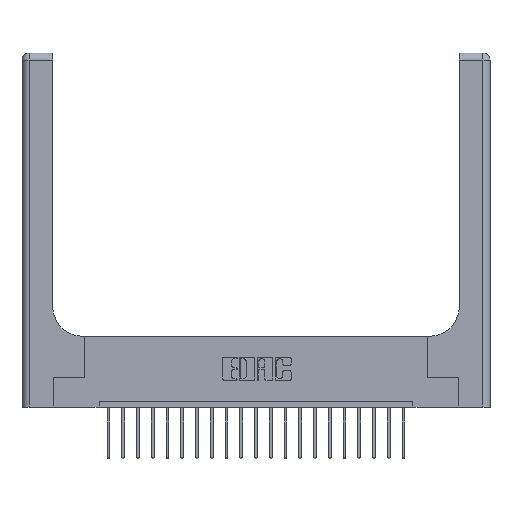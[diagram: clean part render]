
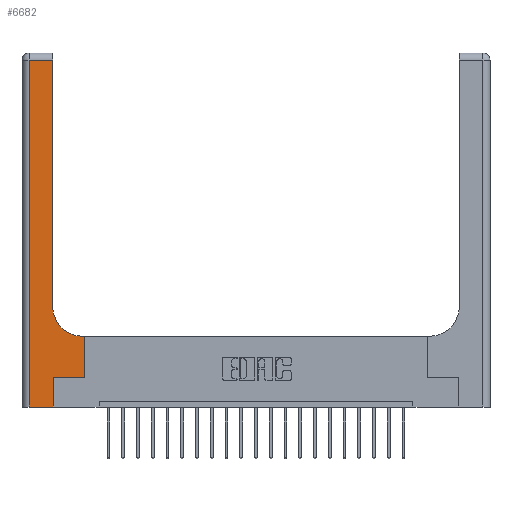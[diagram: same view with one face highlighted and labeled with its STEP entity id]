
A CAD part, top view. The second image highlights one B-rep face of the part: STEP entity #6682.
In plain terms, the highlighted planar face has unit normal (0, 0, 1).
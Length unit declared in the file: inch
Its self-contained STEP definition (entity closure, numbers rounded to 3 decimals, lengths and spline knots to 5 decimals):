
#1258 = DIRECTION ( 'NONE',  ( 0., 0., -1. ) ) ;
#1287 = EDGE_CURVE ( 'NONE', #20009, #4010, #11198, .T. ) ;
#1305 = VERTEX_POINT ( 'NONE', #16613 ) ;
#1809 = EDGE_CURVE ( 'NONE', #7656, #2058, #10814, .T. ) ;
#2058 = VERTEX_POINT ( 'NONE', #15242 ) ;
#2691 = PLANE ( 'NONE',  #3644 ) ;
#2785 = ORIENTED_EDGE ( 'NONE', *, *, #13702, .T. ) ;
#3242 = DIRECTION ( 'NONE',  ( 0., -1., 0. ) ) ;
#3540 = CARTESIAN_POINT ( 'NONE',  ( 0.265, 0.25, 0.37 ) ) ;
#3644 = AXIS2_PLACEMENT_3D ( 'NONE', #16156, #1258, #12577 ) ;
#4010 = VERTEX_POINT ( 'NONE', #3540 ) ;
#4066 = VECTOR ( 'NONE', #6361, 39.37008 ) ;
#4165 = CARTESIAN_POINT ( 'NONE',  ( 0.265, 0.25, 0.37 ) ) ;
#4568 = CARTESIAN_POINT ( 'NONE',  ( 0., 0., 0.37 ) ) ;
#4676 = LINE ( 'NONE', #4568, #19640 ) ;
#4828 = EDGE_CURVE ( 'NONE', #13716, #13617, #13362, .T. ) ;
#5092 = CARTESIAN_POINT ( 'NONE',  ( 0., 2.94, 0.37 ) ) ;
#5202 = CIRCLE ( 'NONE', #13519, 0.25 ) ;
#5622 = DIRECTION ( 'NONE',  ( -1., 0., 0. ) ) ;
#5660 = CARTESIAN_POINT ( 'NONE',  ( 0.528, 0.6, 0.37 ) ) ;
#5676 = DIRECTION ( 'NONE',  ( 1., 0., 0. ) ) ;
#5829 = FACE_OUTER_BOUND ( 'NONE', #11002, .T. ) ;
#6361 = DIRECTION ( 'NONE',  ( 0., 1., 0. ) ) ;
#6502 = VECTOR ( 'NONE', #21473, 39.37008 ) ;
#6559 = DIRECTION ( 'NONE',  ( 1., 0., 0. ) ) ;
#6682 = ADVANCED_FACE ( 'NONE', ( #5829 ), #2691, .F. ) ;
#6691 = LINE ( 'NONE', #14870, #6502 ) ;
#6918 = CARTESIAN_POINT ( 'NONE',  ( 0.265, 0., 0.37 ) ) ;
#7656 = VERTEX_POINT ( 'NONE', #5660 ) ;
#8380 = ORIENTED_EDGE ( 'NONE', *, *, #20369, .T. ) ;
#8544 = ORIENTED_EDGE ( 'NONE', *, *, #10698, .T. ) ;
#8976 = ORIENTED_EDGE ( 'NONE', *, *, #1287, .T. ) ;
#9119 = VECTOR ( 'NONE', #5622, 39.37008 ) ;
#9152 = VECTOR ( 'NONE', #5676, 39.37008 ) ;
#10463 = ORIENTED_EDGE ( 'NONE', *, *, #15314, .T. ) ;
#10698 = EDGE_CURVE ( 'NONE', #13617, #1305, #19646, .T. ) ;
#10814 = LINE ( 'NONE', #17547, #13255 ) ;
#11002 = EDGE_LOOP ( 'NONE', ( #14235, #15795, #8544, #13313, #8976, #2785, #8380, #20760, #10463 ) ) ;
#11198 = LINE ( 'NONE', #17822, #12829 ) ;
#11212 = DIRECTION ( 'NONE',  ( 1., 0., 0. ) ) ;
#11392 = CARTESIAN_POINT ( 'NONE',  ( 0.06, 3., 0.37 ) ) ;
#11993 = CARTESIAN_POINT ( 'NONE',  ( 0.26, 0.85, 0.37 ) ) ;
#12577 = DIRECTION ( 'NONE',  ( -1., 0., 0. ) ) ;
#12829 = VECTOR ( 'NONE', #16188, 39.37008 ) ;
#13099 = CARTESIAN_POINT ( 'NONE',  ( 0.51, 0.85, 0.37 ) ) ;
#13255 = VECTOR ( 'NONE', #14290, 39.37008 ) ;
#13313 = ORIENTED_EDGE ( 'NONE', *, *, #19430, .T. ) ;
#13330 = CARTESIAN_POINT ( 'NONE',  ( 0.528, 0.25, 0.37 ) ) ;
#13362 = LINE ( 'NONE', #5092, #9119 ) ;
#13518 = CARTESIAN_POINT ( 'NONE',  ( 0.06, 2.94, 0.37 ) ) ;
#13519 = AXIS2_PLACEMENT_3D ( 'NONE', #13099, #21232, #6559 ) ;
#13617 = VERTEX_POINT ( 'NONE', #13518 ) ;
#13702 = EDGE_CURVE ( 'NONE', #4010, #19165, #18628, .T. ) ;
#13716 = VERTEX_POINT ( 'NONE', #17097 ) ;
#13845 = VERTEX_POINT ( 'NONE', #11993 ) ;
#14235 = ORIENTED_EDGE ( 'NONE', *, *, #20728, .T. ) ;
#14279 = VECTOR ( 'NONE', #3242, 39.37008 ) ;
#14290 = DIRECTION ( 'NONE',  ( -1., 0., 0. ) ) ;
#14642 = LINE ( 'NONE', #21249, #4066 ) ;
#14870 = CARTESIAN_POINT ( 'NONE',  ( 0.26, 3., 0.37 ) ) ;
#15242 = CARTESIAN_POINT ( 'NONE',  ( 0.51, 0.6, 0.37 ) ) ;
#15314 = EDGE_CURVE ( 'NONE', #2058, #13845, #5202, .T. ) ;
#15795 = ORIENTED_EDGE ( 'NONE', *, *, #4828, .T. ) ;
#16156 = CARTESIAN_POINT ( 'NONE',  ( 0., 3., 0.37 ) ) ;
#16188 = DIRECTION ( 'NONE',  ( 0., 1., 0. ) ) ;
#16613 = CARTESIAN_POINT ( 'NONE',  ( 0.06, 0., 0.37 ) ) ;
#17097 = CARTESIAN_POINT ( 'NONE',  ( 0.26, 2.94, 0.37 ) ) ;
#17547 = CARTESIAN_POINT ( 'NONE',  ( 0.26, 0.6, 0.37 ) ) ;
#17822 = CARTESIAN_POINT ( 'NONE',  ( 0.265, 0., 0.37 ) ) ;
#18628 = LINE ( 'NONE', #4165, #9152 ) ;
#19165 = VERTEX_POINT ( 'NONE', #13330 ) ;
#19430 = EDGE_CURVE ( 'NONE', #1305, #20009, #4676, .T. ) ;
#19640 = VECTOR ( 'NONE', #11212, 39.37008 ) ;
#19646 = LINE ( 'NONE', #11392, #14279 ) ;
#20009 = VERTEX_POINT ( 'NONE', #6918 ) ;
#20369 = EDGE_CURVE ( 'NONE', #19165, #7656, #14642, .T. ) ;
#20728 = EDGE_CURVE ( 'NONE', #13845, #13716, #6691, .T. ) ;
#20760 = ORIENTED_EDGE ( 'NONE', *, *, #1809, .T. ) ;
#21232 = DIRECTION ( 'NONE',  ( 0., 0., -1. ) ) ;
#21249 = CARTESIAN_POINT ( 'NONE',  ( 0.528, 0.25, 0.37 ) ) ;
#21473 = DIRECTION ( 'NONE',  ( 0., 1., 0. ) ) ;
